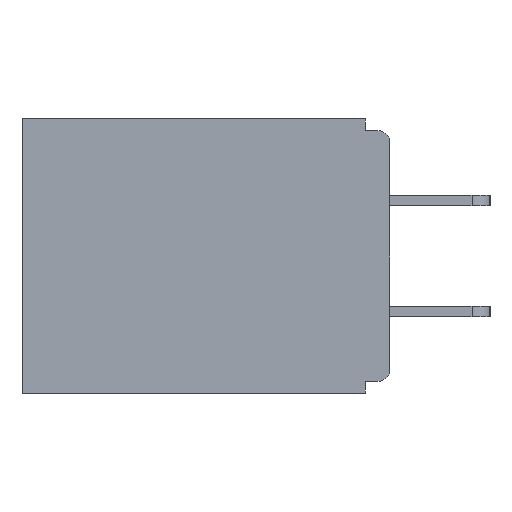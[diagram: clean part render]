
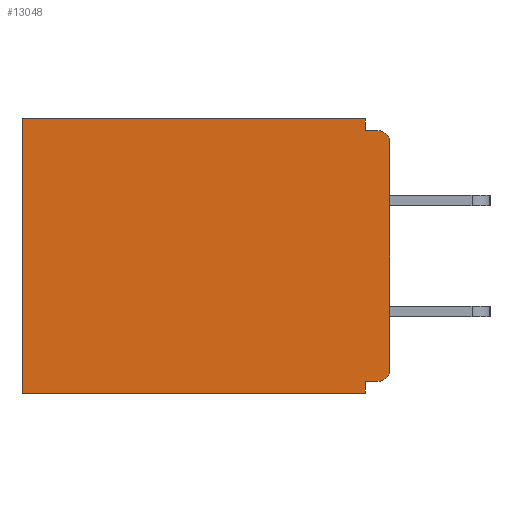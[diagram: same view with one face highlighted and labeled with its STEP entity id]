
A CAD part, left-side view. The second image highlights one B-rep face of the part: STEP entity #13048.
In plain terms, the highlighted planar face has unit normal (-1, 0, 0).
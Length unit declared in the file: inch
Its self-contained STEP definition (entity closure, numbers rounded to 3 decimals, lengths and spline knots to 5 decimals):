
#136 = CARTESIAN_POINT ( 'NONE',  ( 0.298, 0.031, -0.328 ) ) ;
#395 = CARTESIAN_POINT ( 'NONE',  ( 0.298, 0.46, 0. ) ) ;
#510 = ORIENTED_EDGE ( 'NONE', *, *, #4301, .T. ) ;
#853 = LINE ( 'NONE', #17040, #13987 ) ;
#1284 = ORIENTED_EDGE ( 'NONE', *, *, #3620, .T. ) ;
#1308 = VERTEX_POINT ( 'NONE', #8928 ) ;
#1637 = FACE_OUTER_BOUND ( 'NONE', #17533, .T. ) ;
#1769 = EDGE_CURVE ( 'NONE', #17540, #5295, #7909, .T. ) ;
#2602 = VERTEX_POINT ( 'NONE', #16103 ) ;
#2812 = VECTOR ( 'NONE', #11045, 39.37008 ) ;
#2854 = DIRECTION ( 'NONE',  ( 1., 0., 0. ) ) ;
#2873 = DIRECTION ( 'NONE',  ( 0., 1., 0. ) ) ;
#3210 = VECTOR ( 'NONE', #8146, 39.37008 ) ;
#3476 = CARTESIAN_POINT ( 'NONE',  ( 0.298, 0., -0.313 ) ) ;
#3620 = EDGE_CURVE ( 'NONE', #7706, #9746, #13816, .T. ) ;
#3729 = LINE ( 'NONE', #9097, #10509 ) ;
#3917 = CIRCLE ( 'NONE', #4573, 0.015 ) ;
#4154 = VECTOR ( 'NONE', #2873, 39.37008 ) ;
#4301 = EDGE_CURVE ( 'NONE', #2602, #17540, #6972, .T. ) ;
#4335 = LINE ( 'NONE', #5505, #2812 ) ;
#4573 = AXIS2_PLACEMENT_3D ( 'NONE', #6571, #16254, #10771 ) ;
#5270 = CARTESIAN_POINT ( 'NONE',  ( 0.298, 0.46, 0. ) ) ;
#5295 = VERTEX_POINT ( 'NONE', #17371 ) ;
#5334 = CARTESIAN_POINT ( 'NONE',  ( 0.298, 0.015, -0.03 ) ) ;
#5336 = LINE ( 'NONE', #8588, #5769 ) ;
#5505 = CARTESIAN_POINT ( 'NONE',  ( 0.298, 0., -0.328 ) ) ;
#5769 = VECTOR ( 'NONE', #12707, 39.37008 ) ;
#6013 = DIRECTION ( 'NONE',  ( 0., -1., 0. ) ) ;
#6571 = CARTESIAN_POINT ( 'NONE',  ( 0.298, 0.015, -0.313 ) ) ;
#6868 = CARTESIAN_POINT ( 'NONE',  ( 0.298, 0.031, -0.343 ) ) ;
#6972 = LINE ( 'NONE', #9781, #4154 ) ;
#7706 = VERTEX_POINT ( 'NONE', #17454 ) ;
#7909 = LINE ( 'NONE', #5270, #12337 ) ;
#7928 = ORIENTED_EDGE ( 'NONE', *, *, #10794, .T. ) ;
#8146 = DIRECTION ( 'NONE',  ( 0., 0., -1. ) ) ;
#8243 = VECTOR ( 'NONE', #9767, 39.37008 ) ;
#8253 = DIRECTION ( 'NONE',  ( -1., 0., 0. ) ) ;
#8386 = ORIENTED_EDGE ( 'NONE', *, *, #12079, .F. ) ;
#8588 = CARTESIAN_POINT ( 'NONE',  ( 0.298, 0., -0.343 ) ) ;
#8604 = VERTEX_POINT ( 'NONE', #15754 ) ;
#8769 = ORIENTED_EDGE ( 'NONE', *, *, #13019, .F. ) ;
#8928 = CARTESIAN_POINT ( 'NONE',  ( 0.298, 0.031, -0.343 ) ) ;
#9097 = CARTESIAN_POINT ( 'NONE',  ( 0.298, 0., 0. ) ) ;
#9421 = AXIS2_PLACEMENT_3D ( 'NONE', #15547, #2854, #16981 ) ;
#9746 = VERTEX_POINT ( 'NONE', #15459 ) ;
#9767 = DIRECTION ( 'NONE',  ( 0., 0., -1. ) ) ;
#9781 = CARTESIAN_POINT ( 'NONE',  ( 0.298, 0., 0. ) ) ;
#10017 = EDGE_CURVE ( 'NONE', #7706, #11874, #3729, .T. ) ;
#10112 = ORIENTED_EDGE ( 'NONE', *, *, #11182, .F. ) ;
#10405 = EDGE_CURVE ( 'NONE', #15374, #9746, #853, .T. ) ;
#10509 = VECTOR ( 'NONE', #16315, 39.37008 ) ;
#10771 = DIRECTION ( 'NONE',  ( 0., 0., -1. ) ) ;
#10794 = EDGE_CURVE ( 'NONE', #8604, #11874, #3917, .T. ) ;
#11045 = DIRECTION ( 'NONE',  ( 0., 1., 0. ) ) ;
#11182 = EDGE_CURVE ( 'NONE', #15413, #1308, #11997, .T. ) ;
#11266 = EDGE_CURVE ( 'NONE', #8604, #15413, #4335, .T. ) ;
#11433 = PLANE ( 'NONE',  #9421 ) ;
#11874 = VERTEX_POINT ( 'NONE', #3476 ) ;
#11997 = LINE ( 'NONE', #14353, #8243 ) ;
#12079 = EDGE_CURVE ( 'NONE', #2602, #15374, #17048, .T. ) ;
#12337 = VECTOR ( 'NONE', #16341, 39.37008 ) ;
#12707 = DIRECTION ( 'NONE',  ( 0., 1., 0. ) ) ;
#13019 = EDGE_CURVE ( 'NONE', #1308, #5295, #5336, .T. ) ;
#13048 = ADVANCED_FACE ( 'NONE', ( #1637 ), #11433, .F. ) ;
#13749 = AXIS2_PLACEMENT_3D ( 'NONE', #5334, #8253, #18120 ) ;
#13816 = CIRCLE ( 'NONE', #13749, 0.015 ) ;
#13987 = VECTOR ( 'NONE', #6013, 39.37008 ) ;
#14353 = CARTESIAN_POINT ( 'NONE',  ( 0.298, 0.031, -0.343 ) ) ;
#14554 = ORIENTED_EDGE ( 'NONE', *, *, #1769, .T. ) ;
#14863 = ORIENTED_EDGE ( 'NONE', *, *, #10017, .F. ) ;
#15374 = VERTEX_POINT ( 'NONE', #17055 ) ;
#15413 = VERTEX_POINT ( 'NONE', #136 ) ;
#15459 = CARTESIAN_POINT ( 'NONE',  ( 0.298, 0.015, -0.015 ) ) ;
#15541 = ORIENTED_EDGE ( 'NONE', *, *, #10405, .F. ) ;
#15547 = CARTESIAN_POINT ( 'NONE',  ( 0.298, 0., 0. ) ) ;
#15754 = CARTESIAN_POINT ( 'NONE',  ( 0.298, 0.015, -0.328 ) ) ;
#16103 = CARTESIAN_POINT ( 'NONE',  ( 0.298, 0.031, 0. ) ) ;
#16254 = DIRECTION ( 'NONE',  ( -1., 0., 0. ) ) ;
#16315 = DIRECTION ( 'NONE',  ( 0., 0., -1. ) ) ;
#16341 = DIRECTION ( 'NONE',  ( 0., 0., -1. ) ) ;
#16981 = DIRECTION ( 'NONE',  ( 0., 0., -1. ) ) ;
#17040 = CARTESIAN_POINT ( 'NONE',  ( 0.298, 0., -0.015 ) ) ;
#17048 = LINE ( 'NONE', #6868, #3210 ) ;
#17055 = CARTESIAN_POINT ( 'NONE',  ( 0.298, 0.031, -0.015 ) ) ;
#17371 = CARTESIAN_POINT ( 'NONE',  ( 0.298, 0.46, -0.343 ) ) ;
#17454 = CARTESIAN_POINT ( 'NONE',  ( 0.298, 0., -0.03 ) ) ;
#17533 = EDGE_LOOP ( 'NONE', ( #1284, #15541, #8386, #510, #14554, #8769, #10112, #18113, #7928, #14863 ) ) ;
#17540 = VERTEX_POINT ( 'NONE', #395 ) ;
#18113 = ORIENTED_EDGE ( 'NONE', *, *, #11266, .F. ) ;
#18120 = DIRECTION ( 'NONE',  ( 0., 0., -1. ) ) ;
